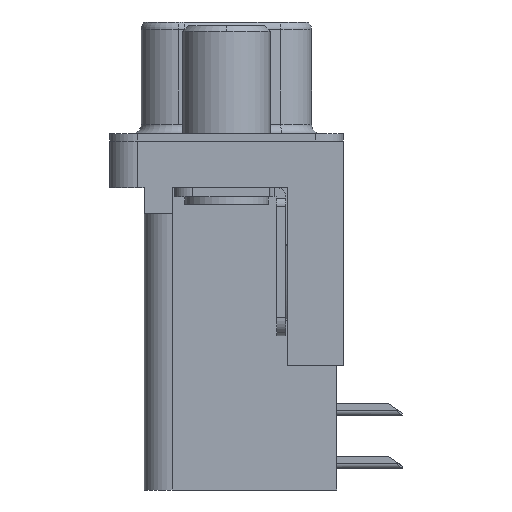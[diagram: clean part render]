
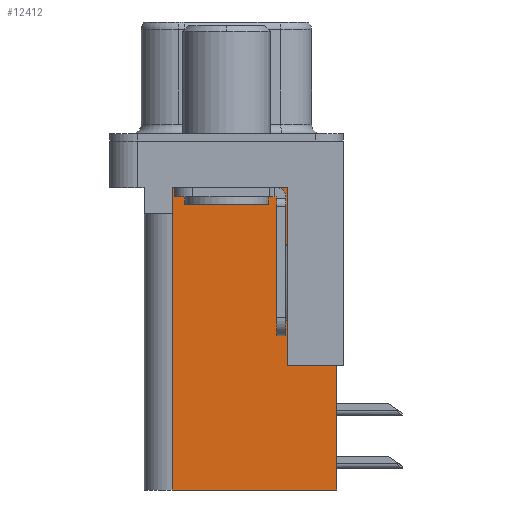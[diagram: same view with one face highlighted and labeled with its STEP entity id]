
A CAD part, left-side view. The second image highlights one B-rep face of the part: STEP entity #12412.
In plain terms, the highlighted planar face has unit normal (-1, 0, 0).
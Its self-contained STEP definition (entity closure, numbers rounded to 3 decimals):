
#114 = EDGE_CURVE ( 'NONE', #4233, #13405, #14069, .T. ) ;
#979 = CARTESIAN_POINT ( 'NONE',  ( 3.79, 2.925, -3.9 ) ) ;
#1191 = VECTOR ( 'NONE', #15740, 1000. ) ;
#1227 = CARTESIAN_POINT ( 'NONE',  ( 3.79, -3.295, -18.76 ) ) ;
#2689 = ORIENTED_EDGE ( 'NONE', *, *, #6743, .T. ) ;
#2787 = CARTESIAN_POINT ( 'NONE',  ( 3.79, -5.925, -18.76 ) ) ;
#3008 = ORIENTED_EDGE ( 'NONE', *, *, #5423, .T. ) ;
#3041 = ORIENTED_EDGE ( 'NONE', *, *, #10340, .F. ) ;
#3096 = CARTESIAN_POINT ( 'NONE',  ( 3.79, 2.895, -3.9 ) ) ;
#3273 = LINE ( 'NONE', #13914, #7100 ) ;
#3589 = PLANE ( 'NONE',  #8729 ) ;
#4017 = CARTESIAN_POINT ( 'NONE',  ( 3.79, 2.925, -18.76 ) ) ;
#4233 = VERTEX_POINT ( 'NONE', #9914 ) ;
#4399 = DIRECTION ( 'NONE',  ( 0., 1., 0. ) ) ;
#4778 = DIRECTION ( 'NONE',  ( 0., 1., 0. ) ) ;
#4944 = LINE ( 'NONE', #8631, #1191 ) ;
#5033 = CARTESIAN_POINT ( 'NONE',  ( 3.79, -3.295, -18.76 ) ) ;
#5423 = EDGE_CURVE ( 'NONE', #17713, #14608, #3273, .T. ) ;
#5556 = LINE ( 'NONE', #16145, #12644 ) ;
#5616 = CARTESIAN_POINT ( 'NONE',  ( 3.79, -3.295, -2.5 ) ) ;
#5669 = EDGE_CURVE ( 'NONE', #14608, #11762, #11502, .T. ) ;
#6101 = VECTOR ( 'NONE', #15539, 1000. ) ;
#6743 = EDGE_CURVE ( 'NONE', #13405, #17713, #16551, .T. ) ;
#6918 = ORIENTED_EDGE ( 'NONE', *, *, #114, .T. ) ;
#6981 = FACE_OUTER_BOUND ( 'NONE', #8144, .T. ) ;
#7100 = VECTOR ( 'NONE', #15334, 1000. ) ;
#7317 = VECTOR ( 'NONE', #4399, 1000. ) ;
#8144 = EDGE_LOOP ( 'NONE', ( #2689, #3008, #16195, #3041, #11982, #12352, #11285, #6918 ) ) ;
#8631 = CARTESIAN_POINT ( 'NONE',  ( 3.79, -5.925, -2. ) ) ;
#8725 = CARTESIAN_POINT ( 'NONE',  ( 3.79, -3.295, -2.5 ) ) ;
#8729 = AXIS2_PLACEMENT_3D ( 'NONE', #5033, #17784, #9313 ) ;
#9313 = DIRECTION ( 'NONE',  ( 0., 1., 0. ) ) ;
#9914 = CARTESIAN_POINT ( 'NONE',  ( 3.79, -3.295, -12.05 ) ) ;
#10090 = CARTESIAN_POINT ( 'NONE',  ( 3.79, 2.925, -18.76 ) ) ;
#10091 = VECTOR ( 'NONE', #15351, 1000. ) ;
#10340 = EDGE_CURVE ( 'NONE', #11150, #11762, #18316, .T. ) ;
#10359 = VECTOR ( 'NONE', #15787, 1000. ) ;
#11150 = VERTEX_POINT ( 'NONE', #4017 ) ;
#11285 = ORIENTED_EDGE ( 'NONE', *, *, #14742, .T. ) ;
#11502 = LINE ( 'NONE', #17160, #7317 ) ;
#11563 = DIRECTION ( 'NONE',  ( 0., 1., 0. ) ) ;
#11762 = VERTEX_POINT ( 'NONE', #979 ) ;
#11877 = EDGE_CURVE ( 'NONE', #16424, #11150, #17596, .T. ) ;
#11982 = ORIENTED_EDGE ( 'NONE', *, *, #11877, .F. ) ;
#12352 = ORIENTED_EDGE ( 'NONE', *, *, #12831, .F. ) ;
#12412 = ADVANCED_FACE ( 'NONE', ( #6981 ), #3589, .F. ) ;
#12644 = VECTOR ( 'NONE', #4778, 1000. ) ;
#12831 = EDGE_CURVE ( 'NONE', #14142, #16424, #4944, .T. ) ;
#13066 = CARTESIAN_POINT ( 'NONE',  ( 3.79, -3.295, -18.76 ) ) ;
#13405 = VERTEX_POINT ( 'NONE', #5616 ) ;
#13914 = CARTESIAN_POINT ( 'NONE',  ( 3.79, 2.895, -3.9 ) ) ;
#14069 = LINE ( 'NONE', #13066, #6101 ) ;
#14142 = VERTEX_POINT ( 'NONE', #18212 ) ;
#14608 = VERTEX_POINT ( 'NONE', #3096 ) ;
#14742 = EDGE_CURVE ( 'NONE', #14142, #4233, #5556, .T. ) ;
#15334 = DIRECTION ( 'NONE',  ( 0., 0., -1. ) ) ;
#15351 = DIRECTION ( 'NONE',  ( 0., 1., 0. ) ) ;
#15539 = DIRECTION ( 'NONE',  ( 0., 0., 1. ) ) ;
#15740 = DIRECTION ( 'NONE',  ( 0., 0., -1. ) ) ;
#15787 = DIRECTION ( 'NONE',  ( 0., 0., 1. ) ) ;
#16135 = VECTOR ( 'NONE', #11563, 1000. ) ;
#16145 = CARTESIAN_POINT ( 'NONE',  ( 3.79, -6.295, -12.05 ) ) ;
#16195 = ORIENTED_EDGE ( 'NONE', *, *, #5669, .T. ) ;
#16424 = VERTEX_POINT ( 'NONE', #2787 ) ;
#16551 = LINE ( 'NONE', #8725, #16135 ) ;
#17160 = CARTESIAN_POINT ( 'NONE',  ( 3.79, 0., -3.9 ) ) ;
#17596 = LINE ( 'NONE', #1227, #10091 ) ;
#17713 = VERTEX_POINT ( 'NONE', #18024 ) ;
#17784 = DIRECTION ( 'NONE',  ( 1., 0., 0. ) ) ;
#18024 = CARTESIAN_POINT ( 'NONE',  ( 3.79, 2.895, -2.5 ) ) ;
#18212 = CARTESIAN_POINT ( 'NONE',  ( 3.79, -5.925, -12.05 ) ) ;
#18316 = LINE ( 'NONE', #10090, #10359 ) ;
